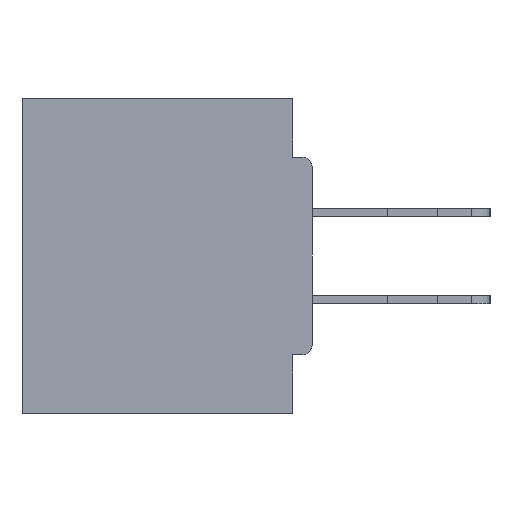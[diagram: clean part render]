
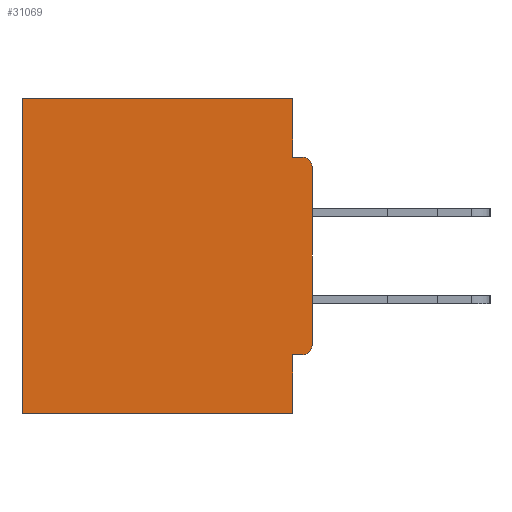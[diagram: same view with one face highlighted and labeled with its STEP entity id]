
A CAD part, left-side view. The second image highlights one B-rep face of the part: STEP entity #31069.
In plain terms, the highlighted planar face has unit normal (-1, 0, 0).
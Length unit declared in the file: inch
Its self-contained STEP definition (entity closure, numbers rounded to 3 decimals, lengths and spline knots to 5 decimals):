
#362 = DIRECTION ( 'NONE',  ( 0., -1., 0. ) ) ;
#620 = CARTESIAN_POINT ( 'NONE',  ( 0.298, 0., -0.0935 ) ) ;
#690 = VERTEX_POINT ( 'NONE', #8846 ) ;
#1018 = LINE ( 'NONE', #35534, #1958 ) ;
#1192 = AXIS2_PLACEMENT_3D ( 'NONE', #12149, #5111, #4594 ) ;
#1237 = DIRECTION ( 'NONE',  ( 0., 0., -1. ) ) ;
#1958 = VECTOR ( 'NONE', #17766, 39.37008 ) ;
#2014 = LINE ( 'NONE', #34334, #37291 ) ;
#2099 = EDGE_CURVE ( 'NONE', #35460, #2454, #34881, .T. ) ;
#2427 = VERTEX_POINT ( 'NONE', #23493 ) ;
#2454 = VERTEX_POINT ( 'NONE', #26692 ) ;
#4342 = CARTESIAN_POINT ( 'NONE',  ( 0.298, 0.015, -0.4065 ) ) ;
#4594 = DIRECTION ( 'NONE',  ( 0., 0., -1. ) ) ;
#4618 = EDGE_CURVE ( 'NONE', #28210, #16128, #25366, .T. ) ;
#5111 = DIRECTION ( 'NONE',  ( 1., 0., 0. ) ) ;
#5845 = DIRECTION ( 'NONE',  ( 0., 0., -1. ) ) ;
#5853 = LINE ( 'NONE', #28070, #22998 ) ;
#6068 = EDGE_LOOP ( 'NONE', ( #14679, #10466, #18522, #24365, #32039, #11567, #11624, #27470, #23560, #10810 ) ) ;
#6541 = EDGE_CURVE ( 'NONE', #38293, #28210, #5853, .T. ) ;
#6845 = VECTOR ( 'NONE', #5845, 39.37008 ) ;
#6889 = FACE_OUTER_BOUND ( 'NONE', #6068, .T. ) ;
#7037 = EDGE_CURVE ( 'NONE', #2427, #35940, #21614, .T. ) ;
#7173 = DIRECTION ( 'NONE',  ( 0., 0., -1. ) ) ;
#7791 = EDGE_CURVE ( 'NONE', #690, #35940, #24763, .T. ) ;
#7873 = DIRECTION ( 'NONE',  ( 0., 0., -1. ) ) ;
#8347 = CIRCLE ( 'NONE', #34068, 0.015 ) ;
#8404 = EDGE_CURVE ( 'NONE', #38293, #2427, #20542, .T. ) ;
#8846 = CARTESIAN_POINT ( 'NONE',  ( 0.298, 0.031, -0.5 ) ) ;
#10306 = CARTESIAN_POINT ( 'NONE',  ( 0.298, 0.46, 0. ) ) ;
#10315 = AXIS2_PLACEMENT_3D ( 'NONE', #10991, #10496, #7873 ) ;
#10466 = ORIENTED_EDGE ( 'NONE', *, *, #4618, .F. ) ;
#10496 = DIRECTION ( 'NONE',  ( -1., 0., 0. ) ) ;
#10810 = ORIENTED_EDGE ( 'NONE', *, *, #25183, .F. ) ;
#10991 = CARTESIAN_POINT ( 'NONE',  ( 0.298, 0.015, -0.3915 ) ) ;
#11567 = ORIENTED_EDGE ( 'NONE', *, *, #7791, .F. ) ;
#11624 = ORIENTED_EDGE ( 'NONE', *, *, #37539, .F. ) ;
#12149 = CARTESIAN_POINT ( 'NONE',  ( 0.298, 0., 0. ) ) ;
#12791 = CARTESIAN_POINT ( 'NONE',  ( 0.298, 0.015, -0.0935 ) ) ;
#13708 = CARTESIAN_POINT ( 'NONE',  ( 0.298, 0.031, -0.0935 ) ) ;
#14108 = DIRECTION ( 'NONE',  ( 0., 0., -1. ) ) ;
#14660 = VECTOR ( 'NONE', #7173, 39.37008 ) ;
#14679 = ORIENTED_EDGE ( 'NONE', *, *, #17152, .T. ) ;
#15802 = VERTEX_POINT ( 'NONE', #23647 ) ;
#16128 = VERTEX_POINT ( 'NONE', #12791 ) ;
#17152 = EDGE_CURVE ( 'NONE', #31828, #16128, #8347, .T. ) ;
#17766 = DIRECTION ( 'NONE',  ( 0., 1., 0. ) ) ;
#17817 = VECTOR ( 'NONE', #36196, 39.37008 ) ;
#18288 = CARTESIAN_POINT ( 'NONE',  ( 0.298, 0., -0.5 ) ) ;
#18522 = ORIENTED_EDGE ( 'NONE', *, *, #6541, .F. ) ;
#19366 = VECTOR ( 'NONE', #362, 39.37008 ) ;
#19394 = DIRECTION ( 'NONE',  ( -1., 0., 0. ) ) ;
#20542 = LINE ( 'NONE', #20549, #24247 ) ;
#20549 = CARTESIAN_POINT ( 'NONE',  ( 0.298, 0., 0. ) ) ;
#21614 = LINE ( 'NONE', #10306, #14660 ) ;
#22998 = VECTOR ( 'NONE', #33260, 39.37008 ) ;
#23493 = CARTESIAN_POINT ( 'NONE',  ( 0.298, 0.46, 0. ) ) ;
#23560 = ORIENTED_EDGE ( 'NONE', *, *, #2099, .T. ) ;
#23647 = CARTESIAN_POINT ( 'NONE',  ( 0.298, 0.031, -0.4065 ) ) ;
#23915 = PLANE ( 'NONE',  #1192 ) ;
#24247 = VECTOR ( 'NONE', #35085, 39.37008 ) ;
#24365 = ORIENTED_EDGE ( 'NONE', *, *, #8404, .T. ) ;
#24556 = CARTESIAN_POINT ( 'NONE',  ( 0.298, 0.031, 0. ) ) ;
#24763 = LINE ( 'NONE', #18288, #17817 ) ;
#25183 = EDGE_CURVE ( 'NONE', #31828, #2454, #2014, .T. ) ;
#25366 = LINE ( 'NONE', #620, #19366 ) ;
#26692 = CARTESIAN_POINT ( 'NONE',  ( 0.298, 0., -0.3915 ) ) ;
#27470 = ORIENTED_EDGE ( 'NONE', *, *, #36485, .F. ) ;
#27806 = CARTESIAN_POINT ( 'NONE',  ( 0.298, 0.015, -0.1085 ) ) ;
#28070 = CARTESIAN_POINT ( 'NONE',  ( 0.298, 0.031, -0.5 ) ) ;
#28210 = VERTEX_POINT ( 'NONE', #13708 ) ;
#29677 = CARTESIAN_POINT ( 'NONE',  ( 0.298, 0.031, -0.5 ) ) ;
#31069 = ADVANCED_FACE ( 'NONE', ( #6889 ), #23915, .F. ) ;
#31828 = VERTEX_POINT ( 'NONE', #32890 ) ;
#32039 = ORIENTED_EDGE ( 'NONE', *, *, #7037, .T. ) ;
#32890 = CARTESIAN_POINT ( 'NONE',  ( 0.298, 0., -0.1085 ) ) ;
#33260 = DIRECTION ( 'NONE',  ( 0., 0., -1. ) ) ;
#34068 = AXIS2_PLACEMENT_3D ( 'NONE', #27806, #19394, #1237 ) ;
#34281 = CARTESIAN_POINT ( 'NONE',  ( 0.298, 0.46, -0.5 ) ) ;
#34334 = CARTESIAN_POINT ( 'NONE',  ( 0.298, 0., 0. ) ) ;
#34881 = CIRCLE ( 'NONE', #10315, 0.015 ) ;
#35085 = DIRECTION ( 'NONE',  ( 0., 1., 0. ) ) ;
#35460 = VERTEX_POINT ( 'NONE', #4342 ) ;
#35534 = CARTESIAN_POINT ( 'NONE',  ( 0.298, 0., -0.4065 ) ) ;
#35940 = VERTEX_POINT ( 'NONE', #34281 ) ;
#36196 = DIRECTION ( 'NONE',  ( 0., 1., 0. ) ) ;
#36485 = EDGE_CURVE ( 'NONE', #35460, #15802, #1018, .T. ) ;
#37291 = VECTOR ( 'NONE', #14108, 39.37008 ) ;
#37468 = LINE ( 'NONE', #29677, #6845 ) ;
#37539 = EDGE_CURVE ( 'NONE', #15802, #690, #37468, .T. ) ;
#38293 = VERTEX_POINT ( 'NONE', #24556 ) ;
